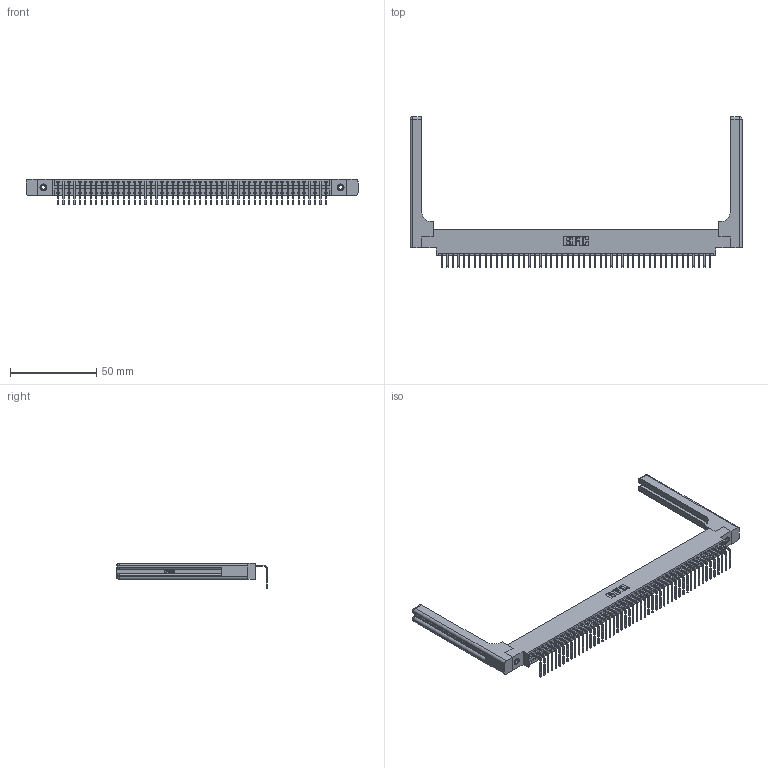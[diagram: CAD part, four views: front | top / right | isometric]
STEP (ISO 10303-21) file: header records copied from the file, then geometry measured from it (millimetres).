
FILE_DESCRIPTION (( 'STEP AP203' ), '1' );
FILE_NAME ('346-050-558-658.STEP', '2022-05-10T04:11:44', ( '' ), ( '' ), 'SwSTEP 2.0', 'SolidWorks 2020', '' );
FILE_SCHEMA (( 'CONFIG_CONTROL_DESIGN' ));
Length unit declared in the file: inch
Products named in the file (5): 346-050-558-658; 345-250-001_345-250-001-102; 346 Part_0.170 Offset - 0.156 Dia-TH; 346-220-058_345-220-058; 345-292-001_558 Tail - 2
Assembly tree (55 placements, depth 2):
  346-050-558-658
    346 Part_0.170 Offset - 0.156 Dia-TH
    345-292-001_558 Tail - 2  x50
    345-250-001_345-250-001-102  x2
    346-220-058_345-220-058  x2
Bounding box: 192.81 x 87.44 x 14.73 mm (x, y, z)
Volume: 26023.7 mm3; surface area: 29571.6 mm2
Topology: 55 solids, 55 shells, 3396 faces, 10143 edges, 6674 vertices
Faces by surface type: plane 2342, cylinder 994, bspline 36, cone 12, sphere 8, torus 4
Entity records: 35768 total; most frequent: CARTESIAN_POINT 7113, ORIENTED_EDGE 5892, DIRECTION 5194, EDGE_CURVE 2946, LINE 2522, VECTOR 2522, VERTEX_POINT 1954, AXIS2_PLACEMENT_3D 1336
